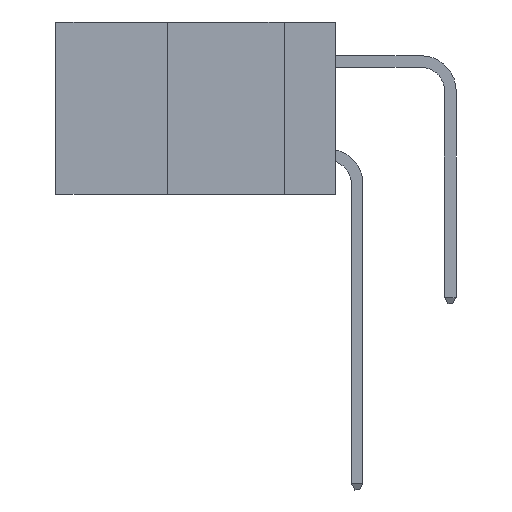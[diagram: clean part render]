
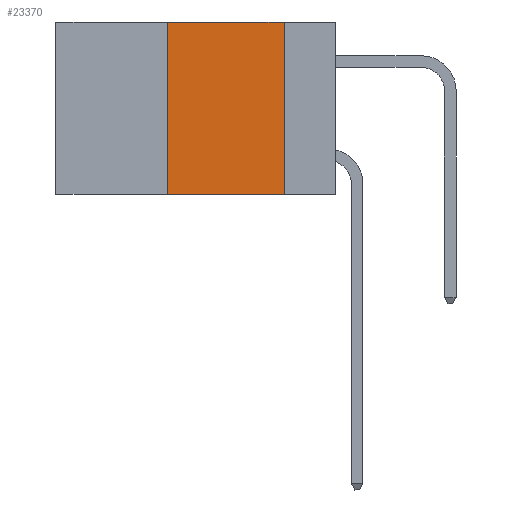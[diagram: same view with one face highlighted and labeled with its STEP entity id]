
A CAD part, left-side view. The second image highlights one B-rep face of the part: STEP entity #23370.
In plain terms, the highlighted planar face has unit normal (-1, 0, 0).
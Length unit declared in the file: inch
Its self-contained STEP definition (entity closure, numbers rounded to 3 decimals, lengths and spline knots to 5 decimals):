
#1703 = ORIENTED_EDGE ( 'NONE', *, *, #31790, .T. ) ;
#1708 = EDGE_CURVE ( 'NONE', #22692, #33234, #41990, .T. ) ;
#2576 = CARTESIAN_POINT ( 'NONE',  ( 0., 0.6, 0. ) ) ;
#2619 = AXIS2_PLACEMENT_3D ( 'NONE', #2978, #22177, #29048 ) ;
#2978 = CARTESIAN_POINT ( 'NONE',  ( 0., 0.6, 0. ) ) ;
#3126 = ORIENTED_EDGE ( 'NONE', *, *, #41394, .F. ) ;
#4012 = CARTESIAN_POINT ( 'NONE',  ( 0., 0.36, 0. ) ) ;
#5628 = LINE ( 'NONE', #33505, #39493 ) ;
#6174 = PLANE ( 'NONE',  #2619 ) ;
#6348 = DIRECTION ( 'NONE',  ( 0., 0., -1. ) ) ;
#7000 = CARTESIAN_POINT ( 'NONE',  ( 0., 0.11, 0. ) ) ;
#10909 = LINE ( 'NONE', #2576, #38524 ) ;
#11757 = VECTOR ( 'NONE', #6348, 39.37008 ) ;
#12085 = DIRECTION ( 'NONE',  ( 0., -1., 0. ) ) ;
#13781 = LINE ( 'NONE', #7000, #11757 ) ;
#18156 = EDGE_LOOP ( 'NONE', ( #3126, #39632, #24779, #1703 ) ) ;
#22177 = DIRECTION ( 'NONE',  ( 1., 0., 0. ) ) ;
#22692 = VERTEX_POINT ( 'NONE', #25803 ) ;
#23370 = ADVANCED_FACE ( 'NONE', ( #24515 ), #6174, .F. ) ;
#24515 = FACE_OUTER_BOUND ( 'NONE', #18156, .T. ) ;
#24779 = ORIENTED_EDGE ( 'NONE', *, *, #1708, .F. ) ;
#25803 = CARTESIAN_POINT ( 'NONE',  ( 0., 0.36, -0.37 ) ) ;
#29014 = VERTEX_POINT ( 'NONE', #38818 ) ;
#29048 = DIRECTION ( 'NONE',  ( 0., 0., -1. ) ) ;
#30323 = DIRECTION ( 'NONE',  ( 0., -1., 0. ) ) ;
#31599 = CARTESIAN_POINT ( 'NONE',  ( 0., 0.36, 0. ) ) ;
#31790 = EDGE_CURVE ( 'NONE', #22692, #29014, #5628, .T. ) ;
#33234 = VERTEX_POINT ( 'NONE', #4012 ) ;
#33357 = VERTEX_POINT ( 'NONE', #34832 ) ;
#33505 = CARTESIAN_POINT ( 'NONE',  ( 0., 0.6, -0.37 ) ) ;
#34832 = CARTESIAN_POINT ( 'NONE',  ( 0., 0.11, 0. ) ) ;
#35220 = DIRECTION ( 'NONE',  ( 0., 0., 1. ) ) ;
#38524 = VECTOR ( 'NONE', #12085, 39.37008 ) ;
#38818 = CARTESIAN_POINT ( 'NONE',  ( 0., 0.11, -0.37 ) ) ;
#39493 = VECTOR ( 'NONE', #30323, 39.37008 ) ;
#39632 = ORIENTED_EDGE ( 'NONE', *, *, #42349, .F. ) ;
#41394 = EDGE_CURVE ( 'NONE', #33357, #29014, #13781, .T. ) ;
#41990 = LINE ( 'NONE', #31599, #42519 ) ;
#42349 = EDGE_CURVE ( 'NONE', #33234, #33357, #10909, .T. ) ;
#42519 = VECTOR ( 'NONE', #35220, 39.37008 ) ;
